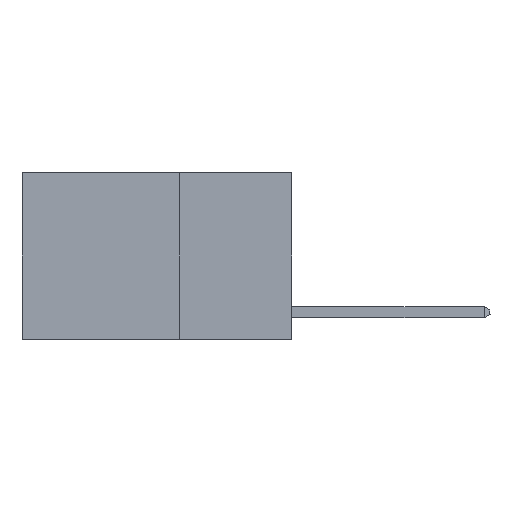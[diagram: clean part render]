
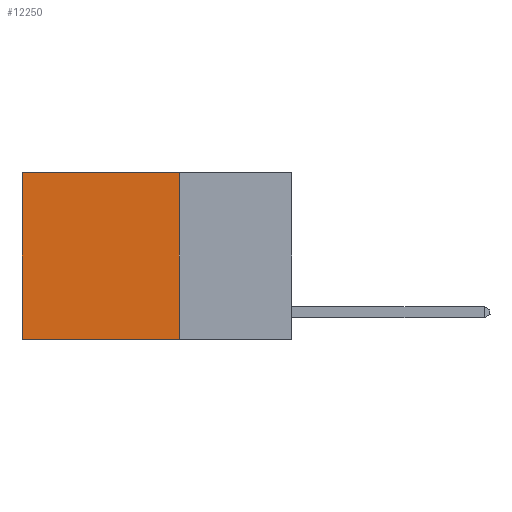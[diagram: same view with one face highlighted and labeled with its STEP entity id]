
A CAD part, left-side view. The second image highlights one B-rep face of the part: STEP entity #12250.
In plain terms, the highlighted planar face has unit normal (-1, 0, 0).
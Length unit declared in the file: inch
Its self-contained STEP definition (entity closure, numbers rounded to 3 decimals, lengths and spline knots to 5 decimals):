
#1088 = LINE ( 'NONE', #6003, #6088 ) ;
#1723 = CARTESIAN_POINT ( 'NONE',  ( 0.2625, 0.6, 0. ) ) ;
#3058 = LINE ( 'NONE', #6823, #8097 ) ;
#3294 = CARTESIAN_POINT ( 'NONE',  ( 0.2625, 0.25, 0. ) ) ;
#4037 = EDGE_CURVE ( 'NONE', #5511, #13608, #1088, .T. ) ;
#5026 = CARTESIAN_POINT ( 'NONE',  ( 0.2625, 0.6, -0.37 ) ) ;
#5499 = ORIENTED_EDGE ( 'NONE', *, *, #4037, .T. ) ;
#5511 = VERTEX_POINT ( 'NONE', #12857 ) ;
#5633 = LINE ( 'NONE', #6827, #9004 ) ;
#5864 = LINE ( 'NONE', #3294, #8043 ) ;
#6003 = CARTESIAN_POINT ( 'NONE',  ( 0.2625, 0.25, 0. ) ) ;
#6088 = VECTOR ( 'NONE', #10864, 39.37008 ) ;
#6763 = VERTEX_POINT ( 'NONE', #11214 ) ;
#6823 = CARTESIAN_POINT ( 'NONE',  ( 0.2625, 0.25, -0.37 ) ) ;
#6827 = CARTESIAN_POINT ( 'NONE',  ( 0.2625, 0.6, 0. ) ) ;
#6874 = EDGE_CURVE ( 'NONE', #6763, #13432, #3058, .T. ) ;
#7635 = EDGE_LOOP ( 'NONE', ( #12717, #11937, #15290, #5499 ) ) ;
#8043 = VECTOR ( 'NONE', #10882, 39.37008 ) ;
#8097 = VECTOR ( 'NONE', #8910, 39.37008 ) ;
#8331 = EDGE_CURVE ( 'NONE', #5511, #6763, #5864, .T. ) ;
#8840 = DIRECTION ( 'NONE',  ( 0., 0., -1. ) ) ;
#8910 = DIRECTION ( 'NONE',  ( 0., 1., 0. ) ) ;
#9004 = VECTOR ( 'NONE', #11682, 39.37008 ) ;
#9408 = EDGE_CURVE ( 'NONE', #13608, #13432, #5633, .T. ) ;
#9653 = PLANE ( 'NONE',  #13878 ) ;
#10864 = DIRECTION ( 'NONE',  ( 0., 1., 0. ) ) ;
#10882 = DIRECTION ( 'NONE',  ( 0., 0., -1. ) ) ;
#11214 = CARTESIAN_POINT ( 'NONE',  ( 0.2625, 0.25, -0.37 ) ) ;
#11682 = DIRECTION ( 'NONE',  ( 0., 0., -1. ) ) ;
#11937 = ORIENTED_EDGE ( 'NONE', *, *, #6874, .F. ) ;
#12250 = ADVANCED_FACE ( 'NONE', ( #15632 ), #9653, .F. ) ;
#12717 = ORIENTED_EDGE ( 'NONE', *, *, #9408, .T. ) ;
#12857 = CARTESIAN_POINT ( 'NONE',  ( 0.2625, 0.25, 0. ) ) ;
#13239 = CARTESIAN_POINT ( 'NONE',  ( 0.2625, 0.25, 0. ) ) ;
#13432 = VERTEX_POINT ( 'NONE', #5026 ) ;
#13608 = VERTEX_POINT ( 'NONE', #1723 ) ;
#13878 = AXIS2_PLACEMENT_3D ( 'NONE', #13239, #14504, #8840 ) ;
#14504 = DIRECTION ( 'NONE',  ( 1., 0., 0. ) ) ;
#15290 = ORIENTED_EDGE ( 'NONE', *, *, #8331, .F. ) ;
#15632 = FACE_OUTER_BOUND ( 'NONE', #7635, .T. ) ;
